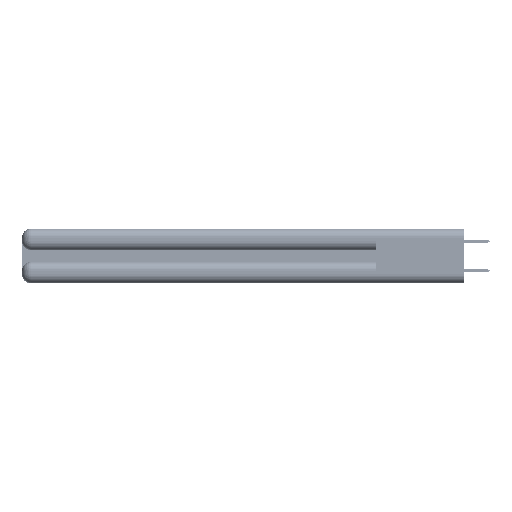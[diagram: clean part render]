
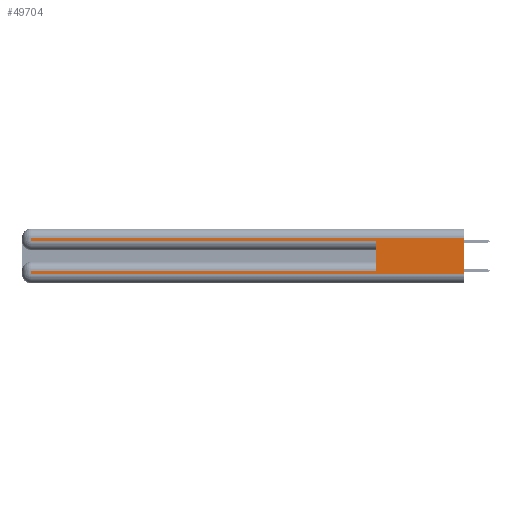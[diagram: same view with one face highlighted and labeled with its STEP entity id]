
A CAD part, left-side view. The second image highlights one B-rep face of the part: STEP entity #49704.
In plain terms, the highlighted planar face has unit normal (-1, 0, 0).
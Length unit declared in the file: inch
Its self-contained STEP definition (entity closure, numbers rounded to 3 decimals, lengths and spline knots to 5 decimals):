
#25 = LINE ( 'NONE', #37148, #31941 ) ;
#966 = VERTEX_POINT ( 'NONE', #21170 ) ;
#1704 = CARTESIAN_POINT ( 'NONE',  ( 0., 0.6, 0.285 ) ) ;
#2824 = CARTESIAN_POINT ( 'NONE',  ( 0., 0., 0.285 ) ) ;
#3206 = ORIENTED_EDGE ( 'NONE', *, *, #29768, .T. ) ;
#3830 = DIRECTION ( 'NONE',  ( 0., 1., 0. ) ) ;
#4293 = PLANE ( 'NONE',  #10613 ) ;
#5283 = DIRECTION ( 'NONE',  ( 0., 0., -1. ) ) ;
#6713 = FACE_OUTER_BOUND ( 'NONE', #8750, .T. ) ;
#7225 = ORIENTED_EDGE ( 'NONE', *, *, #45542, .F. ) ;
#8750 = EDGE_LOOP ( 'NONE', ( #7225, #11793, #46864, #3206, #32627, #20240, #12525, #49813 ) ) ;
#10613 = AXIS2_PLACEMENT_3D ( 'NONE', #21079, #50126, #25258 ) ;
#11506 = EDGE_CURVE ( 'NONE', #48917, #21298, #32382, .T. ) ;
#11793 = ORIENTED_EDGE ( 'NONE', *, *, #25499, .T. ) ;
#11943 = VERTEX_POINT ( 'NONE', #25153 ) ;
#12013 = EDGE_CURVE ( 'NONE', #53236, #966, #40784, .T. ) ;
#12243 = CARTESIAN_POINT ( 'NONE',  ( 0., 2.94, 0.31 ) ) ;
#12525 = ORIENTED_EDGE ( 'NONE', *, *, #41150, .T. ) ;
#14119 = DIRECTION ( 'NONE',  ( 0., 1., 0. ) ) ;
#16333 = EDGE_CURVE ( 'NONE', #38738, #11943, #25, .T. ) ;
#16471 = LINE ( 'NONE', #19809, #46981 ) ;
#17311 = CARTESIAN_POINT ( 'NONE',  ( 0., 2.94, 0.285 ) ) ;
#19802 = LINE ( 'NONE', #27032, #50329 ) ;
#19809 = CARTESIAN_POINT ( 'NONE',  ( 0., 0.6, 0.145 ) ) ;
#20178 = VERTEX_POINT ( 'NONE', #20358 ) ;
#20240 = ORIENTED_EDGE ( 'NONE', *, *, #16333, .T. ) ;
#20270 = LINE ( 'NONE', #26486, #41083 ) ;
#20358 = CARTESIAN_POINT ( 'NONE',  ( 0., 0., 0.31 ) ) ;
#21079 = CARTESIAN_POINT ( 'NONE',  ( 0., 0., 0.37 ) ) ;
#21170 = CARTESIAN_POINT ( 'NONE',  ( 0., 0., 0.06 ) ) ;
#21298 = VERTEX_POINT ( 'NONE', #17311 ) ;
#22452 = VECTOR ( 'NONE', #31958, 39.37008 ) ;
#25153 = CARTESIAN_POINT ( 'NONE',  ( 0., 2.94, 0.085 ) ) ;
#25258 = DIRECTION ( 'NONE',  ( 0., 0., -1. ) ) ;
#25499 = EDGE_CURVE ( 'NONE', #20178, #48917, #20270, .T. ) ;
#26486 = CARTESIAN_POINT ( 'NONE',  ( 0., 0., 0.31 ) ) ;
#27032 = CARTESIAN_POINT ( 'NONE',  ( 0., 2.94, 0.37 ) ) ;
#29752 = VECTOR ( 'NONE', #42217, 39.37008 ) ;
#29768 = EDGE_CURVE ( 'NONE', #21298, #33739, #44587, .T. ) ;
#31941 = VECTOR ( 'NONE', #3830, 39.37008 ) ;
#31958 = DIRECTION ( 'NONE',  ( 0., -1., 0. ) ) ;
#32382 = LINE ( 'NONE', #46597, #53193 ) ;
#32627 = ORIENTED_EDGE ( 'NONE', *, *, #36833, .F. ) ;
#33739 = VERTEX_POINT ( 'NONE', #1704 ) ;
#34232 = DIRECTION ( 'NONE',  ( 0., 0., -1. ) ) ;
#35825 = CARTESIAN_POINT ( 'NONE',  ( 0., 2.94, 0.06 ) ) ;
#36364 = CARTESIAN_POINT ( 'NONE',  ( 0., 0.6, 0.085 ) ) ;
#36833 = EDGE_CURVE ( 'NONE', #38738, #33739, #16471, .T. ) ;
#37148 = CARTESIAN_POINT ( 'NONE',  ( 0., 0., 0.085 ) ) ;
#38738 = VERTEX_POINT ( 'NONE', #36364 ) ;
#40784 = LINE ( 'NONE', #46206, #29752 ) ;
#41083 = VECTOR ( 'NONE', #14119, 39.37008 ) ;
#41150 = EDGE_CURVE ( 'NONE', #11943, #53236, #19802, .T. ) ;
#41722 = VECTOR ( 'NONE', #5283, 39.37008 ) ;
#42217 = DIRECTION ( 'NONE',  ( 0., -1., 0. ) ) ;
#42614 = CARTESIAN_POINT ( 'NONE',  ( 0., 0., 0.37 ) ) ;
#43006 = LINE ( 'NONE', #42614, #41722 ) ;
#43553 = DIRECTION ( 'NONE',  ( 0., 0., -1. ) ) ;
#44587 = LINE ( 'NONE', #2824, #22452 ) ;
#44704 = DIRECTION ( 'NONE',  ( 0., 0., 1. ) ) ;
#45542 = EDGE_CURVE ( 'NONE', #20178, #966, #43006, .T. ) ;
#46206 = CARTESIAN_POINT ( 'NONE',  ( 0., 0., 0.06 ) ) ;
#46597 = CARTESIAN_POINT ( 'NONE',  ( 0., 2.94, 0.37 ) ) ;
#46864 = ORIENTED_EDGE ( 'NONE', *, *, #11506, .T. ) ;
#46981 = VECTOR ( 'NONE', #44704, 39.37008 ) ;
#48917 = VERTEX_POINT ( 'NONE', #12243 ) ;
#49704 = ADVANCED_FACE ( 'NONE', ( #6713 ), #4293, .F. ) ;
#49813 = ORIENTED_EDGE ( 'NONE', *, *, #12013, .T. ) ;
#50126 = DIRECTION ( 'NONE',  ( 1., 0., 0. ) ) ;
#50329 = VECTOR ( 'NONE', #43553, 39.37008 ) ;
#53193 = VECTOR ( 'NONE', #34232, 39.37008 ) ;
#53236 = VERTEX_POINT ( 'NONE', #35825 ) ;
